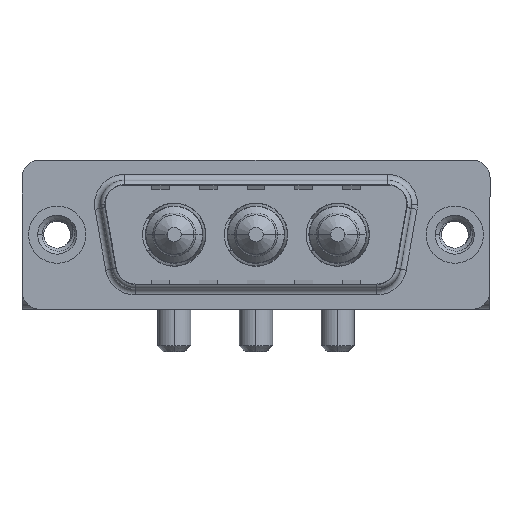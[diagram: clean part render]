
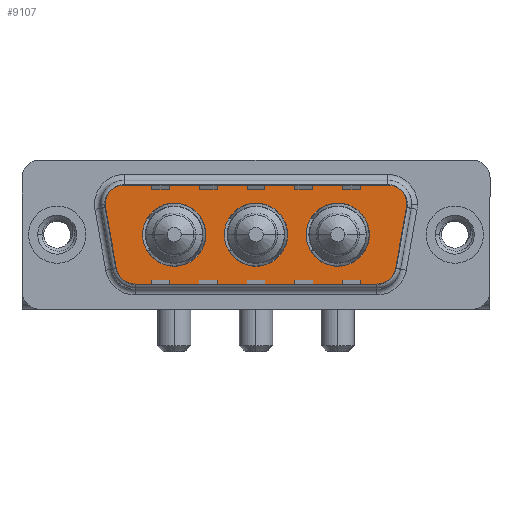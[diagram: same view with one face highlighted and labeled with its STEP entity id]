
A CAD part, top view. The second image highlights one B-rep face of the part: STEP entity #9107.
In plain terms, the highlighted planar face has unit normal (0, 0, 1).
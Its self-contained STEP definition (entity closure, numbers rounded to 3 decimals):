
#357 = CIRCLE ( 'NONE', #8102, 2. ) ;
#391 = CIRCLE ( 'NONE', #2144, 2. ) ;
#462 = EDGE_LOOP ( 'NONE', ( #13511, #4613 ) ) ;
#594 = CIRCLE ( 'NONE', #12709, 2.65 ) ;
#785 = AXIS2_PLACEMENT_3D ( 'NONE', #13181, #5663, #3725 ) ;
#848 = CIRCLE ( 'NONE', #11877, 2. ) ;
#940 = CARTESIAN_POINT ( 'NONE',  ( 6.434, -2.9, 0. ) ) ;
#1194 = CARTESIAN_POINT ( 'NONE',  ( 5.411, 4.9, 0. ) ) ;
#1244 = DIRECTION ( 'NONE',  ( 1., 0., 0. ) ) ;
#1278 = VECTOR ( 'NONE', #7291, 1000. ) ;
#1509 = AXIS2_PLACEMENT_3D ( 'NONE', #1977, #6202, #8418 ) ;
#1518 = FACE_OUTER_BOUND ( 'NONE', #7451, .T. ) ;
#1523 = CARTESIAN_POINT ( 'NONE',  ( 4.464, -3.247, 0. ) ) ;
#1726 = AXIS2_PLACEMENT_3D ( 'NONE', #9556, #2061, #10663 ) ;
#1729 = CARTESIAN_POINT ( 'NONE',  ( 12.45, 0., 0. ) ) ;
#1959 = EDGE_CURVE ( 'NONE', #9565, #6779, #8342, .T. ) ;
#1977 = CARTESIAN_POINT ( 'NONE',  ( 16.65, 0., 0. ) ) ;
#2061 = DIRECTION ( 'NONE',  ( 0., 0., 1. ) ) ;
#2112 = DIRECTION ( 'NONE',  ( 1., 0., 0. ) ) ;
#2144 = AXIS2_PLACEMENT_3D ( 'NONE', #940, #3993, #5291 ) ;
#2306 = DIRECTION ( 'NONE',  ( 1., 0., 0. ) ) ;
#2579 = CIRCLE ( 'NONE', #13600, 2.65 ) ;
#2834 = DIRECTION ( 'NONE',  ( 0., 0., 1. ) ) ;
#2933 = VERTEX_POINT ( 'NONE', #13396 ) ;
#3065 = CARTESIAN_POINT ( 'NONE',  ( 3.441, 2.553, 0. ) ) ;
#3204 = ORIENTED_EDGE ( 'NONE', *, *, #4103, .T. ) ;
#3220 = CARTESIAN_POINT ( 'NONE',  ( 6.434, -4.9, 0. ) ) ;
#3320 = PLANE ( 'NONE',  #5900 ) ;
#3597 = VERTEX_POINT ( 'NONE', #1729 ) ;
#3628 = DIRECTION ( 'NONE',  ( 0., 0., 1. ) ) ;
#3644 = EDGE_CURVE ( 'NONE', #10865, #11497, #3739, .T. ) ;
#3655 = CARTESIAN_POINT ( 'NONE',  ( 19.3, 0., 0. ) ) ;
#3725 = DIRECTION ( 'NONE',  ( -1., 0., 0. ) ) ;
#3739 = CIRCLE ( 'NONE', #1726, 2.65 ) ;
#3833 = CARTESIAN_POINT ( 'NONE',  ( 20.85, 0., 0. ) ) ;
#3881 = VECTOR ( 'NONE', #13016, 1000. ) ;
#3993 = DIRECTION ( 'NONE',  ( 0., 0., 1. ) ) ;
#4103 = EDGE_CURVE ( 'NONE', #11560, #9565, #848, .T. ) ;
#4139 = DIRECTION ( 'NONE',  ( 0., 0., 1. ) ) ;
#4216 = ORIENTED_EDGE ( 'NONE', *, *, #1959, .T. ) ;
#4284 = LINE ( 'NONE', #9492, #6296 ) ;
#4291 = CARTESIAN_POINT ( 'NONE',  ( 26.866, -4.9, 0. ) ) ;
#4321 = CARTESIAN_POINT ( 'NONE',  ( 9.8, 0., 0. ) ) ;
#4433 = ORIENTED_EDGE ( 'NONE', *, *, #7620, .T. ) ;
#4613 = ORIENTED_EDGE ( 'NONE', *, *, #12408, .F. ) ;
#4704 = ORIENTED_EDGE ( 'NONE', *, *, #11291, .F. ) ;
#4741 = EDGE_CURVE ( 'NONE', #4757, #11560, #5417, .T. ) ;
#4757 = VERTEX_POINT ( 'NONE', #13081 ) ;
#5174 = EDGE_CURVE ( 'NONE', #2933, #4757, #5367, .T. ) ;
#5261 = ORIENTED_EDGE ( 'NONE', *, *, #4741, .T. ) ;
#5291 = DIRECTION ( 'NONE',  ( -1., 0., 0. ) ) ;
#5367 = CIRCLE ( 'NONE', #6473, 2. ) ;
#5400 = CARTESIAN_POINT ( 'NONE',  ( 27.889, 2.9, 0. ) ) ;
#5417 = LINE ( 'NONE', #1194, #3881 ) ;
#5465 = VERTEX_POINT ( 'NONE', #3220 ) ;
#5663 = DIRECTION ( 'NONE',  ( 0., 0., 1. ) ) ;
#5666 = ORIENTED_EDGE ( 'NONE', *, *, #5174, .T. ) ;
#5685 = DIRECTION ( 'NONE',  ( 0.174, 0.985, 0. ) ) ;
#5717 = EDGE_CURVE ( 'NONE', #11497, #10865, #12004, .T. ) ;
#5723 = DIRECTION ( 'NONE',  ( 1., 0., 0. ) ) ;
#5749 = CARTESIAN_POINT ( 'NONE',  ( 26.866, -2.9, 0. ) ) ;
#5845 = ORIENTED_EDGE ( 'NONE', *, *, #5717, .F. ) ;
#5900 = AXIS2_PLACEMENT_3D ( 'NONE', #5749, #9987, #1244 ) ;
#5921 = AXIS2_PLACEMENT_3D ( 'NONE', #4321, #10903, #2306 ) ;
#6202 = DIRECTION ( 'NONE',  ( 0., 0., 1. ) ) ;
#6296 = VECTOR ( 'NONE', #13533, 1000. ) ;
#6298 = CIRCLE ( 'NONE', #785, 2. ) ;
#6338 = DIRECTION ( 'NONE',  ( 1., 0., 0. ) ) ;
#6473 = AXIS2_PLACEMENT_3D ( 'NONE', #5400, #9851, #8727 ) ;
#6694 = EDGE_LOOP ( 'NONE', ( #4704, #11181 ) ) ;
#6778 = VERTEX_POINT ( 'NONE', #8047 ) ;
#6779 = VERTEX_POINT ( 'NONE', #1523 ) ;
#6785 = FACE_BOUND ( 'NONE', #462, .T. ) ;
#6816 = CIRCLE ( 'NONE', #1509, 2.65 ) ;
#6821 = DIRECTION ( 'NONE',  ( 1., 0., 0. ) ) ;
#6932 = ORIENTED_EDGE ( 'NONE', *, *, #3644, .F. ) ;
#7151 = AXIS2_PLACEMENT_3D ( 'NONE', #12157, #9817, #5723 ) ;
#7291 = DIRECTION ( 'NONE',  ( 0.174, -0.985, 0. ) ) ;
#7451 = EDGE_LOOP ( 'NONE', ( #12916, #9069, #4433, #5666, #5261, #3204, #4216, #10660, #8041 ) ) ;
#7620 = EDGE_CURVE ( 'NONE', #10485, #2933, #6298, .T. ) ;
#7824 = LINE ( 'NONE', #10818, #12079 ) ;
#7913 = VERTEX_POINT ( 'NONE', #11674 ) ;
#8041 = ORIENTED_EDGE ( 'NONE', *, *, #9330, .T. ) ;
#8047 = CARTESIAN_POINT ( 'NONE',  ( 7.15, 0., 0. ) ) ;
#8096 = DIRECTION ( 'NONE',  ( 1., 0., 0. ) ) ;
#8102 = AXIS2_PLACEMENT_3D ( 'NONE', #9957, #3628, #6821 ) ;
#8342 = LINE ( 'NONE', #3065, #1278 ) ;
#8418 = DIRECTION ( 'NONE',  ( 1., 0., 0. ) ) ;
#8727 = DIRECTION ( 'NONE',  ( -1., 0., 0. ) ) ;
#8940 = EDGE_LOOP ( 'NONE', ( #6932, #5845 ) ) ;
#8986 = CARTESIAN_POINT ( 'NONE',  ( 28.836, -3.247, 0. ) ) ;
#9009 = CIRCLE ( 'NONE', #5921, 2.65 ) ;
#9031 = EDGE_CURVE ( 'NONE', #10029, #10485, #7824, .T. ) ;
#9069 = ORIENTED_EDGE ( 'NONE', *, *, #9031, .T. ) ;
#9107 = ADVANCED_FACE ( 'NONE', ( #6785, #10745, #11023, #1518 ), #3320, .T. ) ;
#9330 = EDGE_CURVE ( 'NONE', #5465, #13457, #4284, .T. ) ;
#9492 = CARTESIAN_POINT ( 'NONE',  ( 6.434, -4.9, 0. ) ) ;
#9556 = CARTESIAN_POINT ( 'NONE',  ( 23.5, 0., 0. ) ) ;
#9565 = VERTEX_POINT ( 'NONE', #12281 ) ;
#9817 = DIRECTION ( 'NONE',  ( 0., 0., 1. ) ) ;
#9851 = DIRECTION ( 'NONE',  ( 0., 0., 1. ) ) ;
#9957 = CARTESIAN_POINT ( 'NONE',  ( 26.866, -2.9, 0. ) ) ;
#9987 = DIRECTION ( 'NONE',  ( 0., 0., 1. ) ) ;
#10029 = VERTEX_POINT ( 'NONE', #8986 ) ;
#10035 = CARTESIAN_POINT ( 'NONE',  ( 29.859, 2.553, 0. ) ) ;
#10110 = EDGE_CURVE ( 'NONE', #6778, #3597, #594, .T. ) ;
#10130 = VERTEX_POINT ( 'NONE', #3655 ) ;
#10161 = EDGE_CURVE ( 'NONE', #13457, #10029, #357, .T. ) ;
#10446 = CARTESIAN_POINT ( 'NONE',  ( 5.411, 2.9, 0. ) ) ;
#10485 = VERTEX_POINT ( 'NONE', #10035 ) ;
#10520 = EDGE_CURVE ( 'NONE', #10130, #7913, #2579, .T. ) ;
#10660 = ORIENTED_EDGE ( 'NONE', *, *, #11118, .T. ) ;
#10663 = DIRECTION ( 'NONE',  ( 1., 0., 0. ) ) ;
#10745 = FACE_BOUND ( 'NONE', #8940, .T. ) ;
#10818 = CARTESIAN_POINT ( 'NONE',  ( 29.859, 2.553, 0. ) ) ;
#10865 = VERTEX_POINT ( 'NONE', #12155 ) ;
#10903 = DIRECTION ( 'NONE',  ( 0., 0., 1. ) ) ;
#11023 = FACE_BOUND ( 'NONE', #6694, .T. ) ;
#11118 = EDGE_CURVE ( 'NONE', #6779, #5465, #391, .T. ) ;
#11181 = ORIENTED_EDGE ( 'NONE', *, *, #10110, .F. ) ;
#11291 = EDGE_CURVE ( 'NONE', #3597, #6778, #9009, .T. ) ;
#11497 = VERTEX_POINT ( 'NONE', #3833 ) ;
#11560 = VERTEX_POINT ( 'NONE', #11572 ) ;
#11572 = CARTESIAN_POINT ( 'NONE',  ( 5.411, 4.9, 0. ) ) ;
#11604 = CARTESIAN_POINT ( 'NONE',  ( 16.65, 0., 0. ) ) ;
#11674 = CARTESIAN_POINT ( 'NONE',  ( 14., 0., 0. ) ) ;
#11877 = AXIS2_PLACEMENT_3D ( 'NONE', #10446, #13655, #2112 ) ;
#12004 = CIRCLE ( 'NONE', #7151, 2.65 ) ;
#12079 = VECTOR ( 'NONE', #5685, 1000. ) ;
#12155 = CARTESIAN_POINT ( 'NONE',  ( 26.15, 0., 0. ) ) ;
#12157 = CARTESIAN_POINT ( 'NONE',  ( 23.5, 0., 0. ) ) ;
#12281 = CARTESIAN_POINT ( 'NONE',  ( 3.441, 2.553, 0. ) ) ;
#12408 = EDGE_CURVE ( 'NONE', #7913, #10130, #6816, .T. ) ;
#12709 = AXIS2_PLACEMENT_3D ( 'NONE', #13258, #2834, #8096 ) ;
#12916 = ORIENTED_EDGE ( 'NONE', *, *, #10161, .T. ) ;
#13016 = DIRECTION ( 'NONE',  ( -1., 0., 0. ) ) ;
#13081 = CARTESIAN_POINT ( 'NONE',  ( 27.889, 4.9, 0. ) ) ;
#13181 = CARTESIAN_POINT ( 'NONE',  ( 27.889, 2.9, 0. ) ) ;
#13258 = CARTESIAN_POINT ( 'NONE',  ( 9.8, 0., 0. ) ) ;
#13396 = CARTESIAN_POINT ( 'NONE',  ( 29.889, 2.9, 0. ) ) ;
#13457 = VERTEX_POINT ( 'NONE', #4291 ) ;
#13511 = ORIENTED_EDGE ( 'NONE', *, *, #10520, .F. ) ;
#13533 = DIRECTION ( 'NONE',  ( 1., 0., 0. ) ) ;
#13600 = AXIS2_PLACEMENT_3D ( 'NONE', #11604, #4139, #6338 ) ;
#13655 = DIRECTION ( 'NONE',  ( 0., 0., 1. ) ) ;
